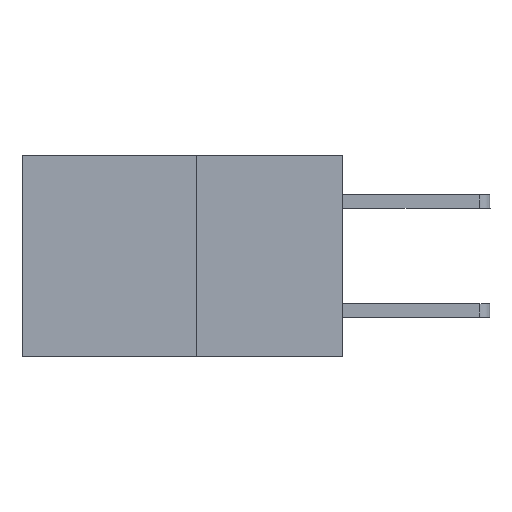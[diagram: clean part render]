
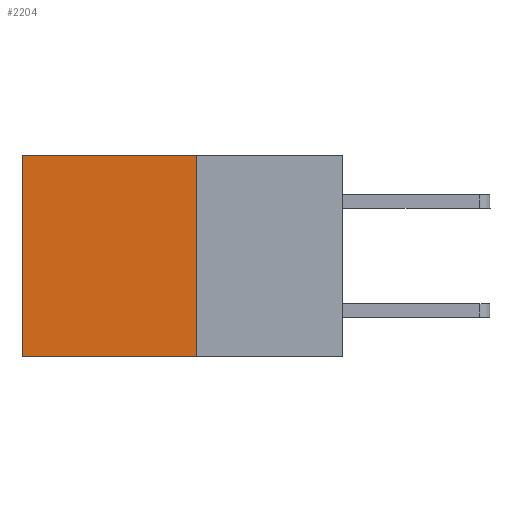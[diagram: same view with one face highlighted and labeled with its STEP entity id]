
A CAD part, left-side view. The second image highlights one B-rep face of the part: STEP entity #2204.
In plain terms, the highlighted planar face has unit normal (-1, 0, 0).
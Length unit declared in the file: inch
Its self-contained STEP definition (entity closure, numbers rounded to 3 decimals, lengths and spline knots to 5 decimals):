
#42 = EDGE_LOOP ( 'NONE', ( #3532, #8964, #8072, #1268 ) ) ;
#146 = VECTOR ( 'NONE', #6210, 39.37008 ) ;
#492 = DIRECTION ( 'NONE',  ( 0., 0., -1. ) ) ;
#600 = VERTEX_POINT ( 'NONE', #8332 ) ;
#746 = EDGE_CURVE ( 'NONE', #4308, #600, #7794, .T. ) ;
#1125 = VECTOR ( 'NONE', #3882, 39.37008 ) ;
#1268 = ORIENTED_EDGE ( 'NONE', *, *, #2686, .T. ) ;
#1464 = CARTESIAN_POINT ( 'NONE',  ( 0.277, 0.27, -0.37 ) ) ;
#2183 = LINE ( 'NONE', #9408, #146 ) ;
#2204 = ADVANCED_FACE ( 'NONE', ( #2433 ), #8119, .F. ) ;
#2284 = EDGE_CURVE ( 'NONE', #3208, #5761, #7543, .T. ) ;
#2433 = FACE_OUTER_BOUND ( 'NONE', #42, .T. ) ;
#2607 = CARTESIAN_POINT ( 'NONE',  ( 0.277, 0.27, 0. ) ) ;
#2686 = EDGE_CURVE ( 'NONE', #3208, #4308, #2183, .T. ) ;
#3208 = VERTEX_POINT ( 'NONE', #2607 ) ;
#3211 = DIRECTION ( 'NONE',  ( 1., 0., 0. ) ) ;
#3223 = CARTESIAN_POINT ( 'NONE',  ( 0.277, 0.59, 0. ) ) ;
#3232 = CARTESIAN_POINT ( 'NONE',  ( 0.277, 0.27, -0.37 ) ) ;
#3532 = ORIENTED_EDGE ( 'NONE', *, *, #746, .T. ) ;
#3882 = DIRECTION ( 'NONE',  ( 0., 1., 0. ) ) ;
#3945 = VECTOR ( 'NONE', #6708, 39.37008 ) ;
#4308 = VERTEX_POINT ( 'NONE', #3223 ) ;
#5285 = LINE ( 'NONE', #6766, #1125 ) ;
#5761 = VERTEX_POINT ( 'NONE', #1464 ) ;
#6210 = DIRECTION ( 'NONE',  ( 0., 1., 0. ) ) ;
#6708 = DIRECTION ( 'NONE',  ( 0., 0., -1. ) ) ;
#6766 = CARTESIAN_POINT ( 'NONE',  ( 0.277, 0.27, -0.37 ) ) ;
#7084 = CARTESIAN_POINT ( 'NONE',  ( 0.277, 0.59, -0.37 ) ) ;
#7543 = LINE ( 'NONE', #8814, #7767 ) ;
#7767 = VECTOR ( 'NONE', #492, 39.37008 ) ;
#7794 = LINE ( 'NONE', #7084, #3945 ) ;
#8072 = ORIENTED_EDGE ( 'NONE', *, *, #2284, .F. ) ;
#8119 = PLANE ( 'NONE',  #8311 ) ;
#8311 = AXIS2_PLACEMENT_3D ( 'NONE', #3232, #3211, #8747 ) ;
#8332 = CARTESIAN_POINT ( 'NONE',  ( 0.277, 0.59, -0.37 ) ) ;
#8747 = DIRECTION ( 'NONE',  ( 0., 0., -1. ) ) ;
#8814 = CARTESIAN_POINT ( 'NONE',  ( 0.277, 0.27, -0.37 ) ) ;
#8857 = EDGE_CURVE ( 'NONE', #5761, #600, #5285, .T. ) ;
#8964 = ORIENTED_EDGE ( 'NONE', *, *, #8857, .F. ) ;
#9408 = CARTESIAN_POINT ( 'NONE',  ( 0.277, 0.27, 0. ) ) ;
